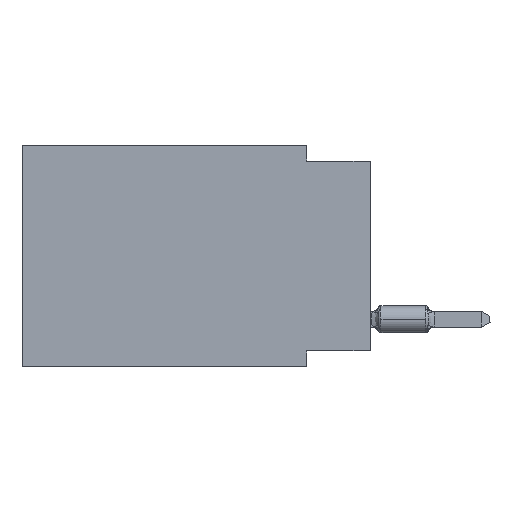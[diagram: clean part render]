
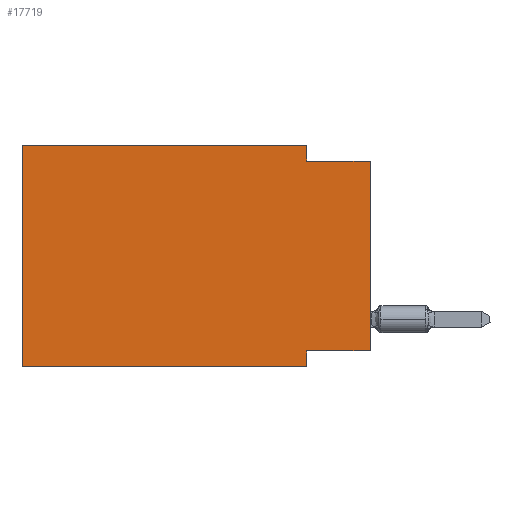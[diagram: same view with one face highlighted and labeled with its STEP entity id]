
A CAD part, left-side view. The second image highlights one B-rep face of the part: STEP entity #17719.
In plain terms, the highlighted planar face has unit normal (-1, 0, 0).
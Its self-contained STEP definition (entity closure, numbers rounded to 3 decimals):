
#80 = LINE ( 'NONE', #2260, #4803 ) ;
#284 = CARTESIAN_POINT ( 'NONE',  ( 0., 2.54, -8.255 ) ) ;
#767 = CARTESIAN_POINT ( 'NONE',  ( 0., 0., 0. ) ) ;
#1145 = DIRECTION ( 'NONE',  ( 0., 0., -1. ) ) ;
#1159 = ORIENTED_EDGE ( 'NONE', *, *, #9377, .F. ) ;
#1402 = ORIENTED_EDGE ( 'NONE', *, *, #26720, .T. ) ;
#1599 = VERTEX_POINT ( 'NONE', #7793 ) ;
#2096 = CARTESIAN_POINT ( 'NONE',  ( 0., 0., -0.635 ) ) ;
#2260 = CARTESIAN_POINT ( 'NONE',  ( 0., 13.97, 0. ) ) ;
#2350 = VECTOR ( 'NONE', #19836, 1000. ) ;
#2604 = EDGE_CURVE ( 'NONE', #10599, #3404, #24383, .T. ) ;
#3146 = CARTESIAN_POINT ( 'NONE',  ( 0., 13.97, 0. ) ) ;
#3309 = CARTESIAN_POINT ( 'NONE',  ( 0., 13.97, 0. ) ) ;
#3404 = VERTEX_POINT ( 'NONE', #23247 ) ;
#4119 = CARTESIAN_POINT ( 'NONE',  ( 0., 2.54, -8.89 ) ) ;
#4145 = VERTEX_POINT ( 'NONE', #19103 ) ;
#4803 = VECTOR ( 'NONE', #23491, 1000. ) ;
#7217 = ORIENTED_EDGE ( 'NONE', *, *, #21127, .F. ) ;
#7428 = VERTEX_POINT ( 'NONE', #29060 ) ;
#7525 = CARTESIAN_POINT ( 'NONE',  ( 0., 2.54, 0. ) ) ;
#7755 = FACE_OUTER_BOUND ( 'NONE', #20765, .T. ) ;
#7793 = CARTESIAN_POINT ( 'NONE',  ( 0., 2.54, -0.635 ) ) ;
#8156 = LINE ( 'NONE', #14615, #30186 ) ;
#8799 = CARTESIAN_POINT ( 'NONE',  ( 0., 0., -8.255 ) ) ;
#8857 = LINE ( 'NONE', #2096, #17937 ) ;
#9097 = AXIS2_PLACEMENT_3D ( 'NONE', #3309, #17130, #1145 ) ;
#9377 = EDGE_CURVE ( 'NONE', #21993, #11742, #18989, .T. ) ;
#10147 = LINE ( 'NONE', #767, #2350 ) ;
#10434 = DIRECTION ( 'NONE',  ( 0., -1., 0. ) ) ;
#10582 = CARTESIAN_POINT ( 'NONE',  ( 0., 13.97, -8.89 ) ) ;
#10599 = VERTEX_POINT ( 'NONE', #26610 ) ;
#11459 = DIRECTION ( 'NONE',  ( 0., 1., 0. ) ) ;
#11460 = DIRECTION ( 'NONE',  ( 0., -1., 0. ) ) ;
#11742 = VERTEX_POINT ( 'NONE', #284 ) ;
#12298 = DIRECTION ( 'NONE',  ( 0., 0., -1. ) ) ;
#12729 = DIRECTION ( 'NONE',  ( 0., 0., -1. ) ) ;
#14615 = CARTESIAN_POINT ( 'NONE',  ( 0., 2.54, -8.89 ) ) ;
#15426 = EDGE_CURVE ( 'NONE', #11742, #22388, #8156, .T. ) ;
#16752 = ORIENTED_EDGE ( 'NONE', *, *, #15426, .F. ) ;
#17130 = DIRECTION ( 'NONE',  ( 1., 0., 0. ) ) ;
#17719 = ADVANCED_FACE ( 'NONE', ( #7755 ), #19450, .F. ) ;
#17937 = VECTOR ( 'NONE', #11460, 1000. ) ;
#18989 = LINE ( 'NONE', #25808, #26055 ) ;
#19103 = CARTESIAN_POINT ( 'NONE',  ( 0., 2.54, 0. ) ) ;
#19316 = ORIENTED_EDGE ( 'NONE', *, *, #2604, .F. ) ;
#19450 = PLANE ( 'NONE',  #9097 ) ;
#19836 = DIRECTION ( 'NONE',  ( 0., 0., 1. ) ) ;
#20765 = EDGE_LOOP ( 'NONE', ( #22589, #21177, #24837, #7217, #19316, #1402, #16752, #1159 ) ) ;
#20963 = EDGE_CURVE ( 'NONE', #21993, #7428, #10147, .T. ) ;
#21127 = EDGE_CURVE ( 'NONE', #3404, #4145, #80, .T. ) ;
#21177 = ORIENTED_EDGE ( 'NONE', *, *, #28488, .F. ) ;
#21993 = VERTEX_POINT ( 'NONE', #8799 ) ;
#22330 = VECTOR ( 'NONE', #12729, 1000. ) ;
#22388 = VERTEX_POINT ( 'NONE', #4119 ) ;
#22589 = ORIENTED_EDGE ( 'NONE', *, *, #20963, .T. ) ;
#23247 = CARTESIAN_POINT ( 'NONE',  ( 0., 13.97, 0. ) ) ;
#23491 = DIRECTION ( 'NONE',  ( 0., -1., 0. ) ) ;
#23665 = VECTOR ( 'NONE', #24536, 1000. ) ;
#24383 = LINE ( 'NONE', #3146, #23665 ) ;
#24536 = DIRECTION ( 'NONE',  ( 0., 0., 1. ) ) ;
#24837 = ORIENTED_EDGE ( 'NONE', *, *, #27862, .F. ) ;
#25244 = VECTOR ( 'NONE', #10434, 1000. ) ;
#25808 = CARTESIAN_POINT ( 'NONE',  ( 0., 0., -8.255 ) ) ;
#26055 = VECTOR ( 'NONE', #11459, 1000. ) ;
#26610 = CARTESIAN_POINT ( 'NONE',  ( 0., 13.97, -8.89 ) ) ;
#26720 = EDGE_CURVE ( 'NONE', #10599, #22388, #27359, .T. ) ;
#27359 = LINE ( 'NONE', #10582, #25244 ) ;
#27862 = EDGE_CURVE ( 'NONE', #4145, #1599, #28615, .T. ) ;
#28488 = EDGE_CURVE ( 'NONE', #1599, #7428, #8857, .T. ) ;
#28615 = LINE ( 'NONE', #7525, #22330 ) ;
#29060 = CARTESIAN_POINT ( 'NONE',  ( 0., 0., -0.635 ) ) ;
#30186 = VECTOR ( 'NONE', #12298, 1000. ) ;
